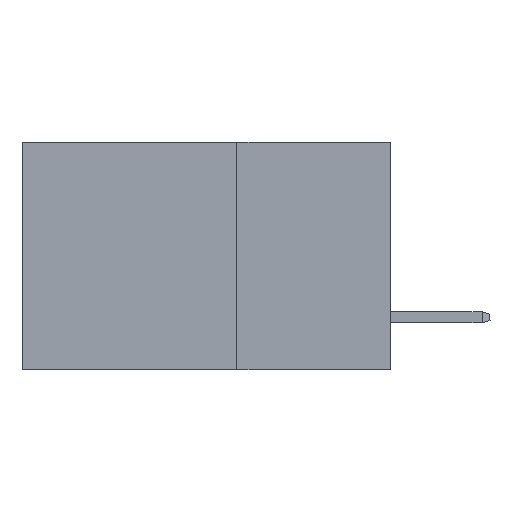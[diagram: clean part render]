
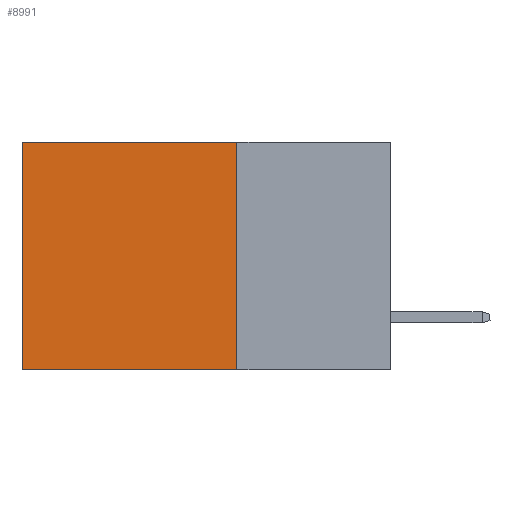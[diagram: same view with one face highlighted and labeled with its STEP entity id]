
A CAD part, left-side view. The second image highlights one B-rep face of the part: STEP entity #8991.
In plain terms, the highlighted planar face has unit normal (-1, 0, 0).
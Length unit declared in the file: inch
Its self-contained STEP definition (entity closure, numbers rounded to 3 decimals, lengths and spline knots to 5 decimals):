
#1204 = PLANE ( 'NONE',  #11763 ) ;
#1321 = VERTEX_POINT ( 'NONE', #17459 ) ;
#2667 = FACE_OUTER_BOUND ( 'NONE', #22642, .T. ) ;
#2745 = VECTOR ( 'NONE', #21751, 39.37008 ) ;
#2848 = VECTOR ( 'NONE', #17936, 39.37008 ) ;
#4935 = ORIENTED_EDGE ( 'NONE', *, *, #17057, .F. ) ;
#5071 = DIRECTION ( 'NONE',  ( 0., 1., 0. ) ) ;
#5478 = LINE ( 'NONE', #14401, #14248 ) ;
#5703 = EDGE_CURVE ( 'NONE', #1321, #22747, #7817, .T. ) ;
#6515 = CARTESIAN_POINT ( 'NONE',  ( 0.2875, 0.6, -0.37 ) ) ;
#6930 = DIRECTION ( 'NONE',  ( 1., 0., 0. ) ) ;
#7817 = LINE ( 'NONE', #16023, #2848 ) ;
#8068 = LINE ( 'NONE', #22076, #17467 ) ;
#8991 = ADVANCED_FACE ( 'NONE', ( #2667 ), #1204, .F. ) ;
#10516 = CARTESIAN_POINT ( 'NONE',  ( 0.2875, 0.25, 0. ) ) ;
#11763 = AXIS2_PLACEMENT_3D ( 'NONE', #18155, #6930, #20030 ) ;
#12114 = EDGE_CURVE ( 'NONE', #12371, #18017, #17959, .T. ) ;
#12371 = VERTEX_POINT ( 'NONE', #20597 ) ;
#13524 = CARTESIAN_POINT ( 'NONE',  ( 0.2875, 0.25, -0.37 ) ) ;
#14248 = VECTOR ( 'NONE', #5071, 39.37008 ) ;
#14401 = CARTESIAN_POINT ( 'NONE',  ( 0.2875, 0.25, -0.37 ) ) ;
#16023 = CARTESIAN_POINT ( 'NONE',  ( 0.2875, 0.6, 0. ) ) ;
#17057 = EDGE_CURVE ( 'NONE', #18017, #22747, #5478, .T. ) ;
#17129 = EDGE_CURVE ( 'NONE', #12371, #1321, #8068, .T. ) ;
#17459 = CARTESIAN_POINT ( 'NONE',  ( 0.2875, 0.6, 0. ) ) ;
#17467 = VECTOR ( 'NONE', #23929, 39.37008 ) ;
#17936 = DIRECTION ( 'NONE',  ( 0., 0., -1. ) ) ;
#17959 = LINE ( 'NONE', #10516, #2745 ) ;
#18017 = VERTEX_POINT ( 'NONE', #13524 ) ;
#18155 = CARTESIAN_POINT ( 'NONE',  ( 0.2875, 0.25, 0. ) ) ;
#19059 = ORIENTED_EDGE ( 'NONE', *, *, #12114, .F. ) ;
#19424 = ORIENTED_EDGE ( 'NONE', *, *, #5703, .T. ) ;
#20030 = DIRECTION ( 'NONE',  ( 0., 0., -1. ) ) ;
#20597 = CARTESIAN_POINT ( 'NONE',  ( 0.2875, 0.25, 0. ) ) ;
#21751 = DIRECTION ( 'NONE',  ( 0., 0., -1. ) ) ;
#22076 = CARTESIAN_POINT ( 'NONE',  ( 0.2875, 0.25, 0. ) ) ;
#22642 = EDGE_LOOP ( 'NONE', ( #19424, #4935, #19059, #24194 ) ) ;
#22747 = VERTEX_POINT ( 'NONE', #6515 ) ;
#23929 = DIRECTION ( 'NONE',  ( 0., 1., 0. ) ) ;
#24194 = ORIENTED_EDGE ( 'NONE', *, *, #17129, .T. ) ;
